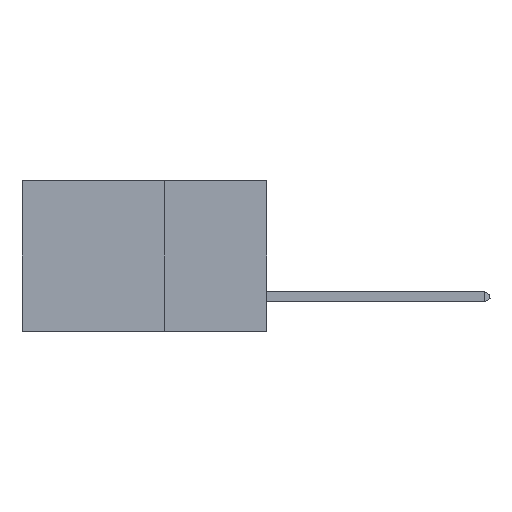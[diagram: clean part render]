
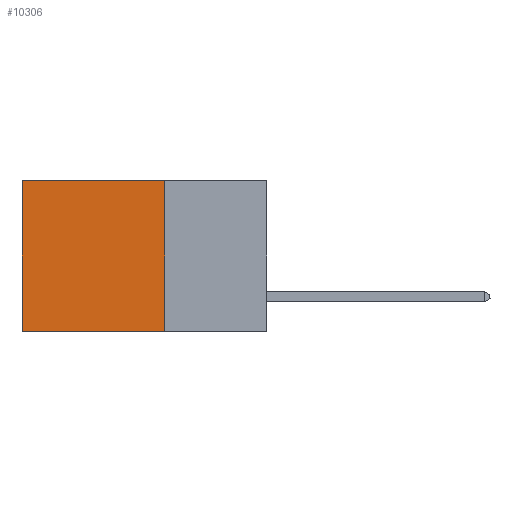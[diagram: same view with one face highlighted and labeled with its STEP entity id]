
A CAD part, left-side view. The second image highlights one B-rep face of the part: STEP entity #10306.
In plain terms, the highlighted planar face has unit normal (-1, 0, 0).
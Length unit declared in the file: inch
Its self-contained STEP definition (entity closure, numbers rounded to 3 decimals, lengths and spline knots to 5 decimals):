
#36 = DIRECTION ( 'NONE',  ( 1., 0., 0. ) ) ;
#556 = EDGE_CURVE ( 'NONE', #7518, #3228, #2255, .T. ) ;
#705 = EDGE_CURVE ( 'NONE', #11289, #3925, #10172, .T. ) ;
#720 = DIRECTION ( 'NONE',  ( 0., 1., 0. ) ) ;
#782 = ORIENTED_EDGE ( 'NONE', *, *, #705, .T. ) ;
#2252 = DIRECTION ( 'NONE',  ( 0., 0., -1. ) ) ;
#2255 = LINE ( 'NONE', #13628, #9355 ) ;
#2301 = VECTOR ( 'NONE', #720, 39.37008 ) ;
#2619 = EDGE_LOOP ( 'NONE', ( #782, #2868, #8883, #12427 ) ) ;
#2868 = ORIENTED_EDGE ( 'NONE', *, *, #12833, .F. ) ;
#3228 = VERTEX_POINT ( 'NONE', #3728 ) ;
#3728 = CARTESIAN_POINT ( 'NONE',  ( 0.2875, 0.25, -0.37 ) ) ;
#3925 = VERTEX_POINT ( 'NONE', #5644 ) ;
#4065 = DIRECTION ( 'NONE',  ( 0., 0., -1. ) ) ;
#4478 = DIRECTION ( 'NONE',  ( 0., 0., -1. ) ) ;
#4642 = FACE_OUTER_BOUND ( 'NONE', #2619, .T. ) ;
#5475 = LINE ( 'NONE', #8843, #9139 ) ;
#5644 = CARTESIAN_POINT ( 'NONE',  ( 0.2875, 0.6, -0.37 ) ) ;
#6331 = CARTESIAN_POINT ( 'NONE',  ( 0.2875, 0.25, 0. ) ) ;
#6733 = DIRECTION ( 'NONE',  ( 0., 1., 0. ) ) ;
#7518 = VERTEX_POINT ( 'NONE', #8020 ) ;
#7535 = EDGE_CURVE ( 'NONE', #7518, #11289, #13064, .T. ) ;
#8020 = CARTESIAN_POINT ( 'NONE',  ( 0.2875, 0.25, 0. ) ) ;
#8843 = CARTESIAN_POINT ( 'NONE',  ( 0.2875, 0.25, -0.37 ) ) ;
#8883 = ORIENTED_EDGE ( 'NONE', *, *, #556, .F. ) ;
#9139 = VECTOR ( 'NONE', #6733, 39.37008 ) ;
#9200 = AXIS2_PLACEMENT_3D ( 'NONE', #6331, #36, #2252 ) ;
#9223 = CARTESIAN_POINT ( 'NONE',  ( 0.2875, 0.6, 0. ) ) ;
#9355 = VECTOR ( 'NONE', #4065, 39.37008 ) ;
#10171 = CARTESIAN_POINT ( 'NONE',  ( 0.2875, 0.25, 0. ) ) ;
#10172 = LINE ( 'NONE', #10980, #10852 ) ;
#10306 = ADVANCED_FACE ( 'NONE', ( #4642 ), #12705, .F. ) ;
#10852 = VECTOR ( 'NONE', #4478, 39.37008 ) ;
#10980 = CARTESIAN_POINT ( 'NONE',  ( 0.2875, 0.6, 0. ) ) ;
#11289 = VERTEX_POINT ( 'NONE', #9223 ) ;
#12427 = ORIENTED_EDGE ( 'NONE', *, *, #7535, .T. ) ;
#12705 = PLANE ( 'NONE',  #9200 ) ;
#12833 = EDGE_CURVE ( 'NONE', #3228, #3925, #5475, .T. ) ;
#13064 = LINE ( 'NONE', #10171, #2301 ) ;
#13628 = CARTESIAN_POINT ( 'NONE',  ( 0.2875, 0.25, 0. ) ) ;
